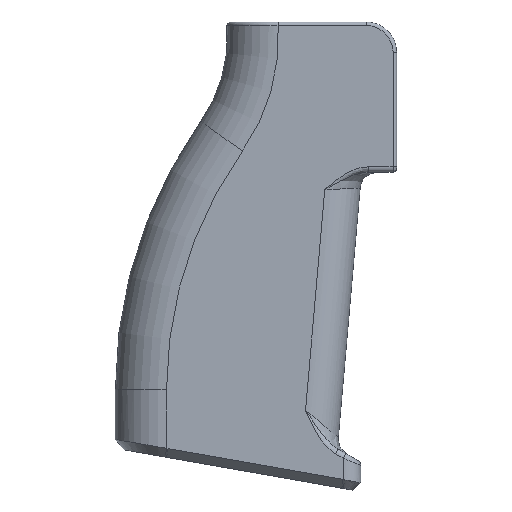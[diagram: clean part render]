
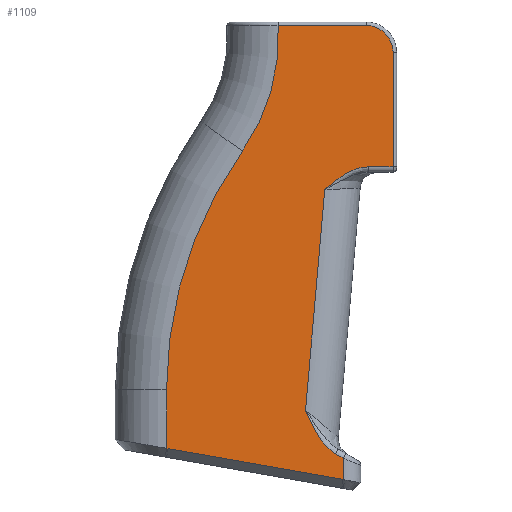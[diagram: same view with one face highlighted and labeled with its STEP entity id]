
A CAD part, left-side view. The second image highlights one B-rep face of the part: STEP entity #1109.
In plain terms, the highlighted planar face has unit normal (-1, 0, 0).
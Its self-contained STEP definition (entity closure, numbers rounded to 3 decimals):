
#49=B_SPLINE_CURVE_WITH_KNOTS('',3,(#2412,#2413,#2414,#2415,#2416,#2417,
#2418,#2419),.UNSPECIFIED.,.F.,.F.,(4,2,1,1,4),(-0.002,0.,
0.7,0.933,1.166),.UNSPECIFIED.);
#50=B_SPLINE_CURVE_WITH_KNOTS('',3,(#2422,#2423,#2424,#2425,#2426,#2427,
#2428,#2429,#2430,#2431,#2432,#2433),.UNSPECIFIED.,.F.,.F.,(4,1,1,1,1,1,
1,2,4),(0.,0.217,0.325,0.434,0.542,
0.65,0.867,1.084,1.085),
 .UNSPECIFIED.);
#81=LINE('',#1583,#163);
#82=LINE('',#1594,#164);
#94=LINE('',#1872,#176);
#137=LINE('',#2319,#219);
#140=LINE('',#2339,#222);
#146=LINE('',#2401,#228);
#147=LINE('',#2408,#229);
#148=LINE('',#2410,#230);
#149=LINE('',#2421,#231);
#163=VECTOR('',#1279,10.);
#164=VECTOR('',#1292,10.);
#176=VECTOR('',#1348,10.);
#219=VECTOR('',#1451,10.);
#222=VECTOR('',#1454,10.);
#228=VECTOR('',#1470,10.);
#229=VECTOR('',#1479,10.);
#230=VECTOR('',#1480,10.);
#231=VECTOR('',#1481,10.);
#308=FACE_OUTER_BOUND('',#380,.T.);
#380=EDGE_LOOP('',(#908,#909,#910,#911,#912,#913,#914,#915,#916,#917,#918,
#919,#920,#921));
#413=CIRCLE('',#1159,5.842);
#442=CIRCLE('',#1222,42.863);
#443=CIRCLE('',#1223,89.884);
#457=VERTEX_POINT('',#1576);
#460=VERTEX_POINT('',#1581);
#462=VERTEX_POINT('',#1586);
#464=VERTEX_POINT('',#1592);
#482=VERTEX_POINT('',#1871);
#522=VERTEX_POINT('',#2146);
#524=VERTEX_POINT('',#2316);
#525=VERTEX_POINT('',#2318);
#533=VERTEX_POINT('',#2400);
#534=VERTEX_POINT('',#2404);
#535=VERTEX_POINT('',#2407);
#536=VERTEX_POINT('',#2409);
#537=VERTEX_POINT('',#2411);
#538=VERTEX_POINT('',#2420);
#560=EDGE_CURVE('',#460,#457,#81,.T.);
#562=EDGE_CURVE('',#462,#460,#413,.T.);
#565=EDGE_CURVE('',#464,#462,#82,.T.);
#594=EDGE_CURVE('',#457,#482,#94,.T.);
#657=EDGE_CURVE('',#524,#525,#137,.T.);
#660=EDGE_CURVE('',#525,#522,#140,.T.);
#672=EDGE_CURVE('',#522,#533,#146,.T.);
#674=EDGE_CURVE('',#534,#464,#442,.T.);
#675=EDGE_CURVE('',#533,#534,#443,.T.);
#676=EDGE_CURVE('',#535,#524,#147,.T.);
#677=EDGE_CURVE('',#536,#535,#148,.T.);
#678=EDGE_CURVE('',#537,#536,#49,.T.);
#679=EDGE_CURVE('',#538,#537,#149,.T.);
#680=EDGE_CURVE('',#482,#538,#50,.T.);
#908=ORIENTED_EDGE('',*,*,#565,.F.);
#909=ORIENTED_EDGE('',*,*,#674,.F.);
#910=ORIENTED_EDGE('',*,*,#675,.F.);
#911=ORIENTED_EDGE('',*,*,#672,.F.);
#912=ORIENTED_EDGE('',*,*,#660,.F.);
#913=ORIENTED_EDGE('',*,*,#657,.F.);
#914=ORIENTED_EDGE('',*,*,#676,.F.);
#915=ORIENTED_EDGE('',*,*,#677,.F.);
#916=ORIENTED_EDGE('',*,*,#678,.F.);
#917=ORIENTED_EDGE('',*,*,#679,.F.);
#918=ORIENTED_EDGE('',*,*,#680,.F.);
#919=ORIENTED_EDGE('',*,*,#594,.F.);
#920=ORIENTED_EDGE('',*,*,#560,.F.);
#921=ORIENTED_EDGE('',*,*,#562,.F.);
#1061=PLANE('',#1221);
#1109=ADVANCED_FACE('',(#308),#1061,.T.);
#1159=AXIS2_PLACEMENT_3D('',#1588,#1284,#1285);
#1221=AXIS2_PLACEMENT_3D('',#2403,#1473,#1474);
#1222=AXIS2_PLACEMENT_3D('',#2405,#1475,#1476);
#1223=AXIS2_PLACEMENT_3D('',#2406,#1477,#1478);
#1279=DIRECTION('',(0.,0.,-1.));
#1284=DIRECTION('center_axis',(1.,0.,0.));
#1285=DIRECTION('ref_axis',(0.,-0.707,0.707));
#1292=DIRECTION('',(0.,-1.,0.));
#1348=DIRECTION('',(0.,1.,0.));
#1451=DIRECTION('',(0.,0.985,0.174));
#1454=DIRECTION('',(0.,0.985,0.174));
#1470=DIRECTION('',(0.,0.,1.));
#1473=DIRECTION('center_axis',(-1.,0.,0.));
#1474=DIRECTION('ref_axis',(0.,-1.,0.));
#1475=DIRECTION('center_axis',(-1.,0.,0.));
#1476=DIRECTION('ref_axis',(0.,-0.968,-0.253));
#1477=DIRECTION('center_axis',(1.,0.,0.));
#1478=DIRECTION('ref_axis',(0.,0.953,0.303));
#1479=DIRECTION('',(0.,0.,-1.));
#1480=DIRECTION('',(0.,-0.866,-0.5));
#1481=DIRECTION('',(0.,0.087,-0.996));
#1576=CARTESIAN_POINT('',(-10.5,9.268,-112.301));
#1581=CARTESIAN_POINT('',(-10.5,9.268,-87.434));
#1583=CARTESIAN_POINT('',(-10.5,9.268,-122.635));
#1586=CARTESIAN_POINT('',(-10.5,15.11,-81.592));
#1588=CARTESIAN_POINT('Origin',(-10.5,15.11,-87.434));
#1592=CARTESIAN_POINT('',(-10.5,34.233,-81.592));
#1594=CARTESIAN_POINT('',(-10.5,27.08,-81.592));
#1871=CARTESIAN_POINT('',(-10.5,14.655,-112.301));
#1872=CARTESIAN_POINT('',(-10.5,27.588,-112.301));
#2146=CARTESIAN_POINT('',(-10.5,58.483,-173.45));
#2316=CARTESIAN_POINT('',(-10.5,20.114,-180.216));
#2318=CARTESIAN_POINT('',(-10.5,58.153,-173.509));
#2319=CARTESIAN_POINT('',(-10.5,58.01,-173.534));
#2339=CARTESIAN_POINT('',(-10.5,58.153,-173.509));
#2400=CARTESIAN_POINT('',(-10.5,58.483,-160.725));
#2401=CARTESIAN_POINT('',(-10.5,58.483,-146.276));
#2403=CARTESIAN_POINT('Origin',(-10.5,39.051,-131.826));
#2404=CARTESIAN_POINT('',(-10.5,42.012,-108.863));
#2405=CARTESIAN_POINT('Origin',(-10.5,77.021,-84.132));
#2406=CARTESIAN_POINT('Origin',(-10.5,-31.401,-160.725));
#2407=CARTESIAN_POINT('',(-10.5,20.114,-175.592));
#2408=CARTESIAN_POINT('',(-10.5,20.114,-157.324));
#2409=CARTESIAN_POINT('',(-10.5,21.776,-174.632));
#2410=CARTESIAN_POINT('',(-10.5,35.071,-166.956));
#2411=CARTESIAN_POINT('',(-10.5,28.298,-165.147));
#2412=CARTESIAN_POINT('Ctrl Pts',(-10.5,28.298,-165.147));
#2413=CARTESIAN_POINT('Ctrl Pts',(-10.5,28.296,-165.152));
#2414=CARTESIAN_POINT('Ctrl Pts',(-10.5,28.294,-165.157));
#2415=CARTESIAN_POINT('Ctrl Pts',(-10.5,27.367,-167.294));
#2416=CARTESIAN_POINT('Ctrl Pts',(-10.5,26.136,-170.21));
#2417=CARTESIAN_POINT('Ctrl Pts',(-10.5,23.689,-173.259));
#2418=CARTESIAN_POINT('Ctrl Pts',(-10.5,22.449,-174.244));
#2419=CARTESIAN_POINT('Ctrl Pts',(-10.5,21.776,-174.632));
#2420=CARTESIAN_POINT('',(-10.5,24.108,-117.254));
#2421=CARTESIAN_POINT('',(-10.5,27.231,-152.944));
#2422=CARTESIAN_POINT('Ctrl Pts',(-10.5,14.655,-112.301));
#2423=CARTESIAN_POINT('Ctrl Pts',(-10.5,15.377,-112.301));
#2424=CARTESIAN_POINT('Ctrl Pts',(-10.5,16.47,-112.464));
#2425=CARTESIAN_POINT('Ctrl Pts',(-10.5,17.846,-112.925));
#2426=CARTESIAN_POINT('Ctrl Pts',(-10.5,18.832,-113.368));
#2427=CARTESIAN_POINT('Ctrl Pts',(-10.5,19.78,-113.895));
#2428=CARTESIAN_POINT('Ctrl Pts',(-10.5,20.999,-114.687));
#2429=CARTESIAN_POINT('Ctrl Pts',(-10.5,22.449,-115.812));
#2430=CARTESIAN_POINT('Ctrl Pts',(-10.5,23.554,-116.772));
#2431=CARTESIAN_POINT('Ctrl Pts',(-10.5,24.102,-117.248));
#2432=CARTESIAN_POINT('Ctrl Pts',(-10.5,24.105,-117.251));
#2433=CARTESIAN_POINT('Ctrl Pts',(-10.5,24.108,-117.254));
